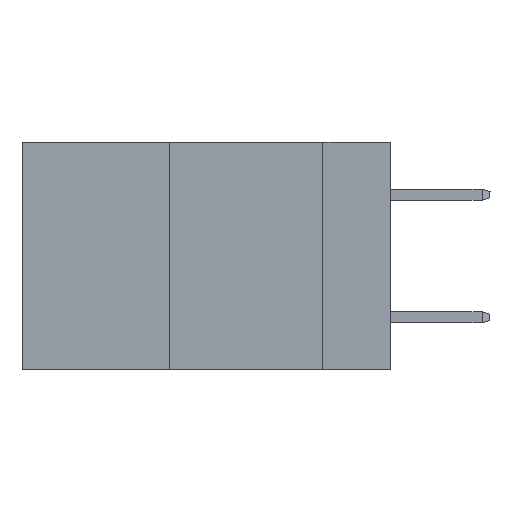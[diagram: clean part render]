
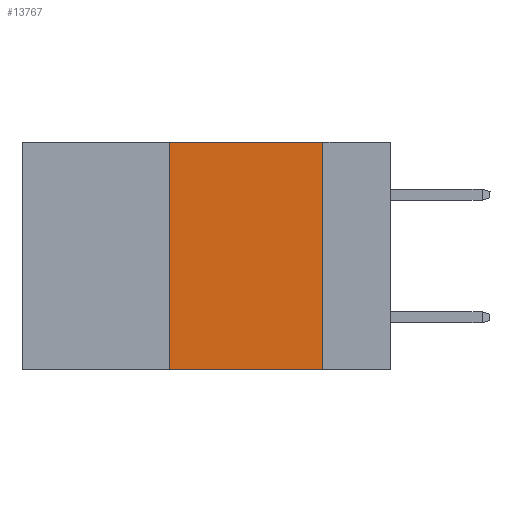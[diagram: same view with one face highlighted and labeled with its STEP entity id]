
A CAD part, left-side view. The second image highlights one B-rep face of the part: STEP entity #13767.
In plain terms, the highlighted planar face has unit normal (-1, 0, 0).
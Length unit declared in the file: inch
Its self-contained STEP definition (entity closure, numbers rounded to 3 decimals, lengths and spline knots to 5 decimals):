
#953 = VERTEX_POINT ( 'NONE', #6867 ) ;
#1371 = PLANE ( 'NONE',  #23773 ) ;
#1479 = DIRECTION ( 'NONE',  ( 0., 0., 1. ) ) ;
#2873 = EDGE_LOOP ( 'NONE', ( #31523, #31671, #10343, #17142 ) ) ;
#3054 = DIRECTION ( 'NONE',  ( 0., 0., -1. ) ) ;
#3565 = FACE_OUTER_BOUND ( 'NONE', #2873, .T. ) ;
#3869 = CARTESIAN_POINT ( 'NONE',  ( 0., 0.11, 0. ) ) ;
#4854 = VECTOR ( 'NONE', #3054, 39.37008 ) ;
#6867 = CARTESIAN_POINT ( 'NONE',  ( 0., 0.36, -0.37 ) ) ;
#7009 = EDGE_CURVE ( 'NONE', #20359, #27292, #11040, .T. ) ;
#7573 = EDGE_CURVE ( 'NONE', #953, #21693, #11826, .T. ) ;
#8723 = DIRECTION ( 'NONE',  ( 0., 0., -1. ) ) ;
#10343 = ORIENTED_EDGE ( 'NONE', *, *, #7573, .F. ) ;
#11040 = LINE ( 'NONE', #26222, #4854 ) ;
#11517 = LINE ( 'NONE', #29361, #23898 ) ;
#11563 = CARTESIAN_POINT ( 'NONE',  ( 0., 0.6, 0. ) ) ;
#11826 = LINE ( 'NONE', #32344, #14940 ) ;
#13188 = CARTESIAN_POINT ( 'NONE',  ( 0., 0.11, -0.37 ) ) ;
#13767 = ADVANCED_FACE ( 'NONE', ( #3565 ), #1371, .F. ) ;
#14365 = DIRECTION ( 'NONE',  ( 0., -1., 0. ) ) ;
#14940 = VECTOR ( 'NONE', #1479, 39.37008 ) ;
#16611 = VECTOR ( 'NONE', #14365, 39.37008 ) ;
#17142 = ORIENTED_EDGE ( 'NONE', *, *, #30169, .T. ) ;
#20359 = VERTEX_POINT ( 'NONE', #3869 ) ;
#21693 = VERTEX_POINT ( 'NONE', #23003 ) ;
#21885 = LINE ( 'NONE', #29549, #16611 ) ;
#23003 = CARTESIAN_POINT ( 'NONE',  ( 0., 0.36, 0. ) ) ;
#23773 = AXIS2_PLACEMENT_3D ( 'NONE', #11563, #23912, #8723 ) ;
#23898 = VECTOR ( 'NONE', #24038, 39.37008 ) ;
#23912 = DIRECTION ( 'NONE',  ( 1., 0., 0. ) ) ;
#24038 = DIRECTION ( 'NONE',  ( 0., -1., 0. ) ) ;
#24568 = EDGE_CURVE ( 'NONE', #21693, #20359, #11517, .T. ) ;
#26222 = CARTESIAN_POINT ( 'NONE',  ( 0., 0.11, 0. ) ) ;
#27292 = VERTEX_POINT ( 'NONE', #13188 ) ;
#29361 = CARTESIAN_POINT ( 'NONE',  ( 0., 0.6, 0. ) ) ;
#29549 = CARTESIAN_POINT ( 'NONE',  ( 0., 0.6, -0.37 ) ) ;
#30169 = EDGE_CURVE ( 'NONE', #953, #27292, #21885, .T. ) ;
#31523 = ORIENTED_EDGE ( 'NONE', *, *, #7009, .F. ) ;
#31671 = ORIENTED_EDGE ( 'NONE', *, *, #24568, .F. ) ;
#32344 = CARTESIAN_POINT ( 'NONE',  ( 0., 0.36, 0. ) ) ;
